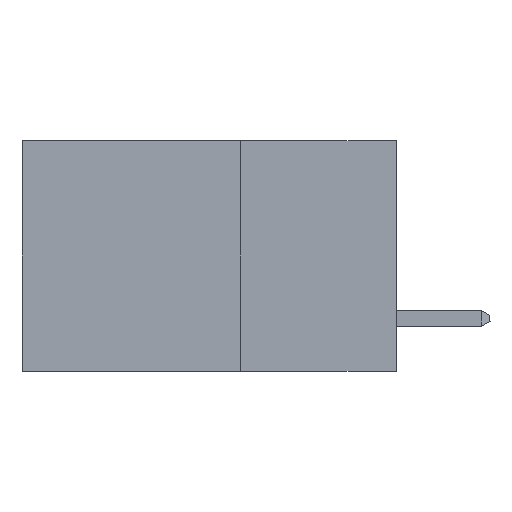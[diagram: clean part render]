
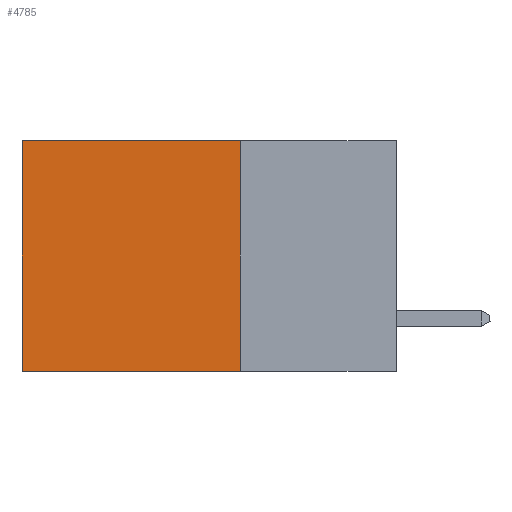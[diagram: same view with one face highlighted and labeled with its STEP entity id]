
A CAD part, left-side view. The second image highlights one B-rep face of the part: STEP entity #4785.
In plain terms, the highlighted planar face has unit normal (-1, 0, 0).
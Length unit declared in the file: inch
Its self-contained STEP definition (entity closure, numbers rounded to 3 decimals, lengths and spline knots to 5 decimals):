
#1306 = LINE ( 'NONE', #16451, #23279 ) ;
#1537 = DIRECTION ( 'NONE',  ( 0., 0., -1. ) ) ;
#1706 = CARTESIAN_POINT ( 'NONE',  ( 0.298, 0.25, -0.37 ) ) ;
#2377 = ORIENTED_EDGE ( 'NONE', *, *, #10541, .T. ) ;
#2901 = ORIENTED_EDGE ( 'NONE', *, *, #16634, .F. ) ;
#4785 = ADVANCED_FACE ( 'NONE', ( #26730 ), #19672, .F. ) ;
#5432 = LINE ( 'NONE', #9833, #7581 ) ;
#5610 = EDGE_CURVE ( 'NONE', #17928, #16872, #5432, .T. ) ;
#6554 = CARTESIAN_POINT ( 'NONE',  ( 0.298, 0.25, 0. ) ) ;
#7485 = ORIENTED_EDGE ( 'NONE', *, *, #5610, .F. ) ;
#7581 = VECTOR ( 'NONE', #16232, 39.37008 ) ;
#8480 = LINE ( 'NONE', #10448, #21218 ) ;
#9833 = CARTESIAN_POINT ( 'NONE',  ( 0.298, 0.25, -0.37 ) ) ;
#10448 = CARTESIAN_POINT ( 'NONE',  ( 0.298, 0.25, 0. ) ) ;
#10541 = EDGE_CURVE ( 'NONE', #28438, #16872, #1306, .T. ) ;
#10737 = AXIS2_PLACEMENT_3D ( 'NONE', #15151, #15047, #1537 ) ;
#15047 = DIRECTION ( 'NONE',  ( 1., 0., 0. ) ) ;
#15151 = CARTESIAN_POINT ( 'NONE',  ( 0.298, 0.25, 0. ) ) ;
#16152 = LINE ( 'NONE', #21839, #23920 ) ;
#16232 = DIRECTION ( 'NONE',  ( 0., 1., 0. ) ) ;
#16451 = CARTESIAN_POINT ( 'NONE',  ( 0.298, 0.6, 0. ) ) ;
#16634 = EDGE_CURVE ( 'NONE', #28276, #17928, #8480, .T. ) ;
#16872 = VERTEX_POINT ( 'NONE', #25059 ) ;
#17037 = DIRECTION ( 'NONE',  ( 0., 0., -1. ) ) ;
#17086 = EDGE_LOOP ( 'NONE', ( #2377, #7485, #2901, #28591 ) ) ;
#17158 = DIRECTION ( 'NONE',  ( 0., 1., 0. ) ) ;
#17928 = VERTEX_POINT ( 'NONE', #1706 ) ;
#18313 = CARTESIAN_POINT ( 'NONE',  ( 0.298, 0.6, 0. ) ) ;
#19672 = PLANE ( 'NONE',  #10737 ) ;
#21218 = VECTOR ( 'NONE', #17037, 39.37008 ) ;
#21839 = CARTESIAN_POINT ( 'NONE',  ( 0.298, 0.25, 0. ) ) ;
#23279 = VECTOR ( 'NONE', #23565, 39.37008 ) ;
#23565 = DIRECTION ( 'NONE',  ( 0., 0., -1. ) ) ;
#23920 = VECTOR ( 'NONE', #17158, 39.37008 ) ;
#25059 = CARTESIAN_POINT ( 'NONE',  ( 0.298, 0.6, -0.37 ) ) ;
#26365 = EDGE_CURVE ( 'NONE', #28276, #28438, #16152, .T. ) ;
#26730 = FACE_OUTER_BOUND ( 'NONE', #17086, .T. ) ;
#28276 = VERTEX_POINT ( 'NONE', #6554 ) ;
#28438 = VERTEX_POINT ( 'NONE', #18313 ) ;
#28591 = ORIENTED_EDGE ( 'NONE', *, *, #26365, .T. ) ;
